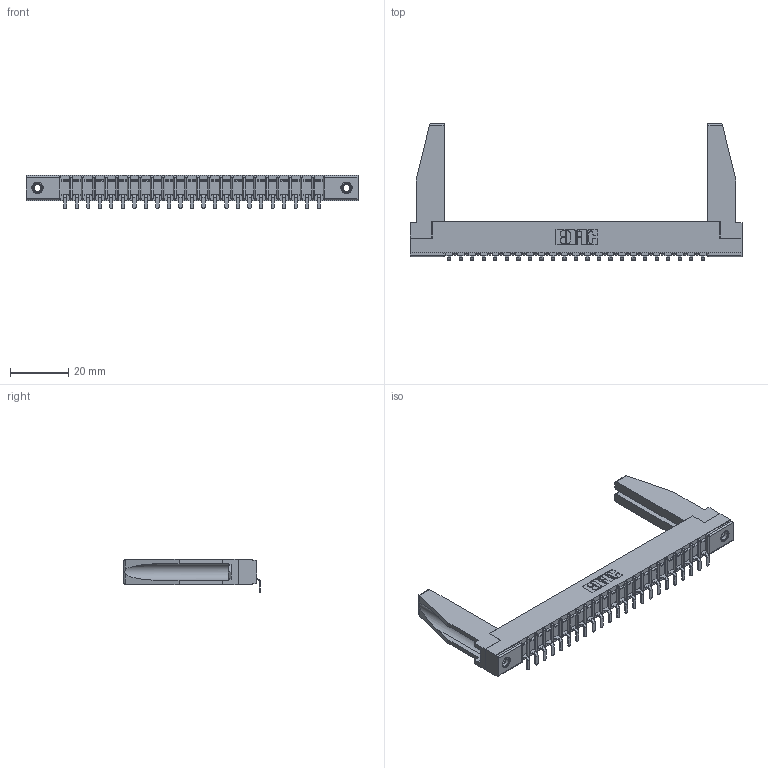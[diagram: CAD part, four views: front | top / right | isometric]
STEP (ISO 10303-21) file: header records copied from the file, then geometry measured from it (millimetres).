
FILE_DESCRIPTION (( 'STEP AP203' ), '1' );
FILE_NAME ('357-023-553-178.STEP', '2019-09-16T23:47:46', ( '' ), ( '' ), 'SwSTEP 2.0', 'SolidWorks 2016', '' );
FILE_SCHEMA (( 'CONFIG_CONTROL_DESIGN' ));
Length unit declared in the file: inch
Products named in the file (5): 307-290-002_553; 357-023-553-178; 307-220-078; 345-250-001_345-250-001-102; 307 Part_.156 Dia Mounting Holes
Assembly tree (28 placements, depth 2):
  357-023-553-178
    307 Part_.156 Dia Mounting Holes
    307-290-002_553  x23
    307-220-078  x2
    345-250-001_345-250-001-102  x2
Bounding box: 114.15 x 47.03 x 11.51 mm (x, y, z)
Volume: 11529.5 mm3; surface area: 17590.5 mm2
Topology: 28 solids, 28 shells, 2066 faces, 6265 edges, 4102 vertices
Faces by surface type: plane 1235, cylinder 767, sphere 48, cone 12, torus 4
Entity records: 25353 total; most frequent: CARTESIAN_POINT 4274, ORIENTED_EDGE 4220, DIRECTION 4118, EDGE_CURVE 2110, LINE 1610, VECTOR 1610, VERTEX_POINT 1368, AXIS2_PLACEMENT_3D 1254
